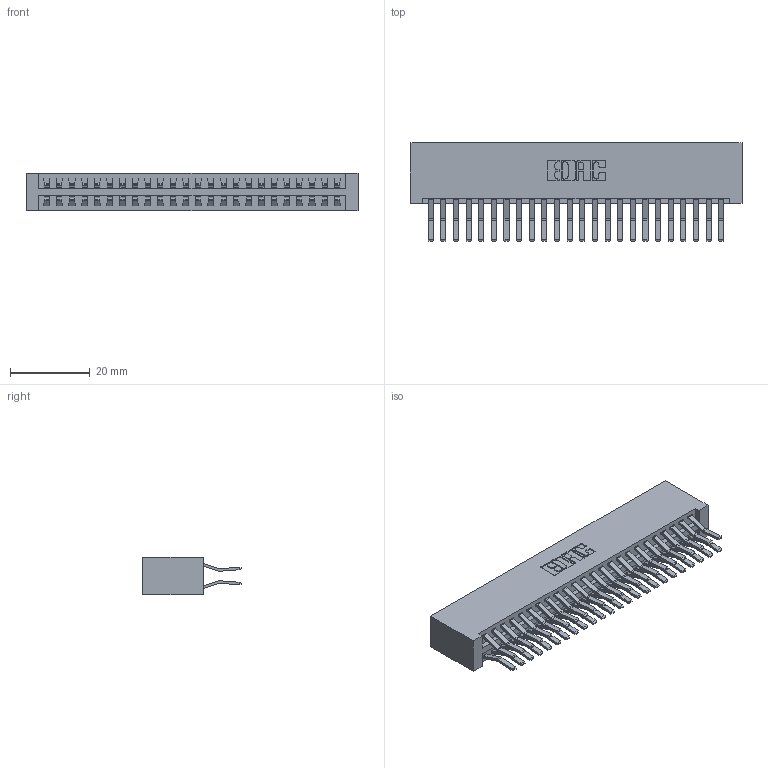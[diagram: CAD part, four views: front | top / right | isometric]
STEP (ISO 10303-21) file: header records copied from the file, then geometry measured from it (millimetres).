
FILE_DESCRIPTION (( 'STEP AP203' ), '1' );
FILE_NAME ('396-048-560-201.STEP', '2018-09-08T01:23:59', ( '' ), ( '' ), 'SwSTEP 2.0', 'SolidWorks 2016', '' );
FILE_SCHEMA (( 'CONFIG_CONTROL_DESIGN' ));
Length unit declared in the file: inch
Products named in the file (3): 346 Part_No Mounting Lugs; 345-292-001_560 Tail; 396-048-560-201
Assembly tree (49 placements, depth 2):
  396-048-560-201
    346 Part_No Mounting Lugs
    345-292-001_560 Tail  x48
Bounding box: 83.44 x 24.78 x 9.4 mm (x, y, z)
Volume: 8884.4 mm3; surface area: 12931.9 mm2
Topology: 49 solids, 49 shells, 2706 faces, 8033 edges, 5290 vertices
Faces by surface type: plane 1752, cylinder 954
Entity records: 17897 total; most frequent: CARTESIAN_POINT 2972, ORIENTED_EDGE 2906, DIRECTION 2669, EDGE_CURVE 1453, LINE 1229, VECTOR 1229, VERTEX_POINT 966, AXIS2_PLACEMENT_3D 720
